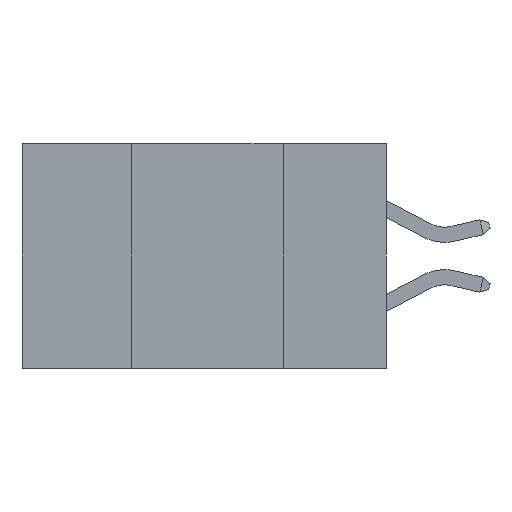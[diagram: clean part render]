
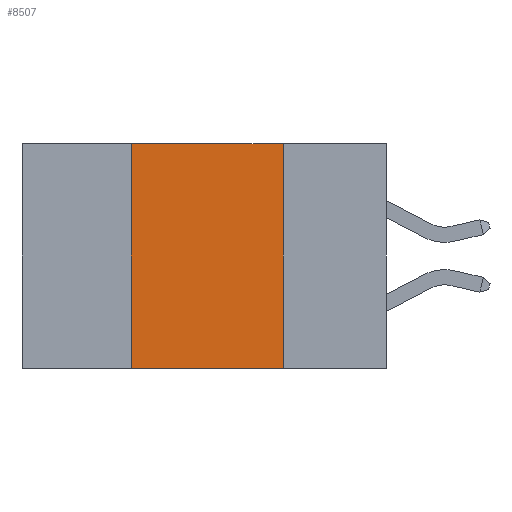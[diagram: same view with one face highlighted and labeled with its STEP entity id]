
A CAD part, left-side view. The second image highlights one B-rep face of the part: STEP entity #8507.
In plain terms, the highlighted planar face has unit normal (-1, 0, 0).
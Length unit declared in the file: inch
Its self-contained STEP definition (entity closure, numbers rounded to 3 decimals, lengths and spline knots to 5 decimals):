
#216 = LINE ( 'NONE', #10111, #2931 ) ;
#656 = CARTESIAN_POINT ( 'NONE',  ( 0., 0.42, -0.37 ) ) ;
#1577 = EDGE_CURVE ( 'NONE', #9669, #8266, #216, .T. ) ;
#2098 = CARTESIAN_POINT ( 'NONE',  ( 0., 0.42, 0. ) ) ;
#2888 = VERTEX_POINT ( 'NONE', #656 ) ;
#2931 = VECTOR ( 'NONE', #3277, 39.37008 ) ;
#2955 = ORIENTED_EDGE ( 'NONE', *, *, #13036, .F. ) ;
#3277 = DIRECTION ( 'NONE',  ( 0., -1., 0. ) ) ;
#3319 = ORIENTED_EDGE ( 'NONE', *, *, #1577, .F. ) ;
#3379 = PLANE ( 'NONE',  #6941 ) ;
#3524 = VERTEX_POINT ( 'NONE', #14777 ) ;
#3729 = CARTESIAN_POINT ( 'NONE',  ( 0., 0.17, 0. ) ) ;
#6315 = LINE ( 'NONE', #2098, #11880 ) ;
#6941 = AXIS2_PLACEMENT_3D ( 'NONE', #12548, #7005, #13693 ) ;
#7005 = DIRECTION ( 'NONE',  ( 1., 0., 0. ) ) ;
#7338 = EDGE_LOOP ( 'NONE', ( #2955, #3319, #10286, #9510 ) ) ;
#7565 = EDGE_CURVE ( 'NONE', #2888, #9669, #6315, .T. ) ;
#7760 = CARTESIAN_POINT ( 'NONE',  ( 0., 0.42, 0. ) ) ;
#8224 = FACE_OUTER_BOUND ( 'NONE', #7338, .T. ) ;
#8266 = VERTEX_POINT ( 'NONE', #13344 ) ;
#8507 = ADVANCED_FACE ( 'NONE', ( #8224 ), #3379, .F. ) ;
#8787 = CARTESIAN_POINT ( 'NONE',  ( 0., 0.6, -0.37 ) ) ;
#9510 = ORIENTED_EDGE ( 'NONE', *, *, #11197, .T. ) ;
#9669 = VERTEX_POINT ( 'NONE', #7760 ) ;
#10111 = CARTESIAN_POINT ( 'NONE',  ( 0., 0.6, 0. ) ) ;
#10286 = ORIENTED_EDGE ( 'NONE', *, *, #7565, .F. ) ;
#10481 = LINE ( 'NONE', #8787, #13161 ) ;
#11197 = EDGE_CURVE ( 'NONE', #2888, #3524, #10481, .T. ) ;
#11880 = VECTOR ( 'NONE', #12436, 39.37008 ) ;
#12317 = DIRECTION ( 'NONE',  ( 0., -1., 0. ) ) ;
#12355 = LINE ( 'NONE', #3729, #14471 ) ;
#12436 = DIRECTION ( 'NONE',  ( 0., 0., 1. ) ) ;
#12548 = CARTESIAN_POINT ( 'NONE',  ( 0., 0.6, 0. ) ) ;
#13036 = EDGE_CURVE ( 'NONE', #8266, #3524, #12355, .T. ) ;
#13161 = VECTOR ( 'NONE', #12317, 39.37008 ) ;
#13344 = CARTESIAN_POINT ( 'NONE',  ( 0., 0.17, 0. ) ) ;
#13693 = DIRECTION ( 'NONE',  ( 0., 0., -1. ) ) ;
#14334 = DIRECTION ( 'NONE',  ( 0., 0., -1. ) ) ;
#14471 = VECTOR ( 'NONE', #14334, 39.37008 ) ;
#14777 = CARTESIAN_POINT ( 'NONE',  ( 0., 0.17, -0.37 ) ) ;
